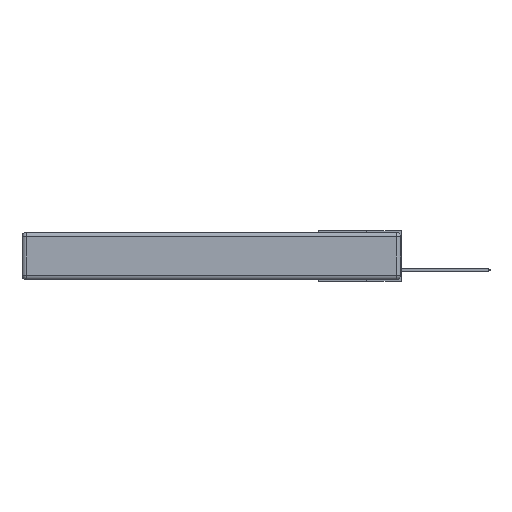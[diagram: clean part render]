
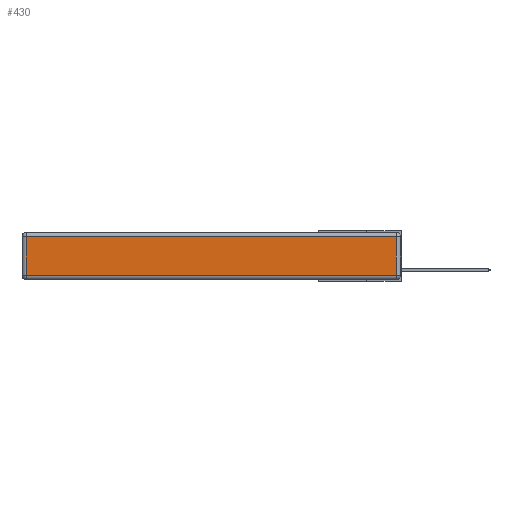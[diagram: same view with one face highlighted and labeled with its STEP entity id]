
A CAD part, left-side view. The second image highlights one B-rep face of the part: STEP entity #430.
In plain terms, the highlighted planar face has unit normal (-1, 0, 0).
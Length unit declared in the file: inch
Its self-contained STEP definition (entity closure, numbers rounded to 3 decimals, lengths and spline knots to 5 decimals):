
#25 = VECTOR ( 'NONE', #13483, 39.37008 ) ;
#243 = CARTESIAN_POINT ( 'NONE',  ( 0., 2.72, -0.343 ) ) ;
#319 = DIRECTION ( 'NONE',  ( 0., 1., 0. ) ) ;
#430 = ADVANCED_FACE ( 'NONE', ( #3738 ), #7658, .T. ) ;
#1101 = ORIENTED_EDGE ( 'NONE', *, *, #12454, .T. ) ;
#1314 = ORIENTED_EDGE ( 'NONE', *, *, #12495, .T. ) ;
#2300 = VERTEX_POINT ( 'NONE', #2312 ) ;
#2312 = CARTESIAN_POINT ( 'NONE',  ( 0., 2.72, -0.03 ) ) ;
#2358 = LINE ( 'NONE', #4114, #3935 ) ;
#2375 = LINE ( 'NONE', #4579, #25 ) ;
#2383 = EDGE_CURVE ( 'NONE', #2300, #3912, #8110, .T. ) ;
#2987 = EDGE_CURVE ( 'NONE', #3912, #9757, #2375, .T. ) ;
#3738 = FACE_OUTER_BOUND ( 'NONE', #11194, .T. ) ;
#3912 = VERTEX_POINT ( 'NONE', #14608 ) ;
#3935 = VECTOR ( 'NONE', #6581, 39.37008 ) ;
#4029 = DIRECTION ( 'NONE',  ( 0., 0., -1. ) ) ;
#4114 = CARTESIAN_POINT ( 'NONE',  ( 0., 0.03, -0.343 ) ) ;
#4579 = CARTESIAN_POINT ( 'NONE',  ( 0., 0., -0.313 ) ) ;
#5947 = VECTOR ( 'NONE', #4029, 39.37008 ) ;
#6581 = DIRECTION ( 'NONE',  ( 0., 0., 1. ) ) ;
#6583 = DIRECTION ( 'NONE',  ( -1., 0., 0. ) ) ;
#7039 = ORIENTED_EDGE ( 'NONE', *, *, #2987, .T. ) ;
#7658 = PLANE ( 'NONE',  #15020 ) ;
#8110 = LINE ( 'NONE', #243, #5947 ) ;
#9052 = CARTESIAN_POINT ( 'NONE',  ( 0., 2.75, -0.03 ) ) ;
#9757 = VERTEX_POINT ( 'NONE', #16175 ) ;
#11194 = EDGE_LOOP ( 'NONE', ( #7039, #1101, #1314, #12809 ) ) ;
#11600 = CARTESIAN_POINT ( 'NONE',  ( 0., 0.03, -0.03 ) ) ;
#11870 = VERTEX_POINT ( 'NONE', #11600 ) ;
#12454 = EDGE_CURVE ( 'NONE', #9757, #11870, #2358, .T. ) ;
#12495 = EDGE_CURVE ( 'NONE', #11870, #2300, #12767, .T. ) ;
#12650 = DIRECTION ( 'NONE',  ( 0., 0., 1. ) ) ;
#12767 = LINE ( 'NONE', #9052, #14311 ) ;
#12775 = CARTESIAN_POINT ( 'NONE',  ( 0., 0., -0.343 ) ) ;
#12809 = ORIENTED_EDGE ( 'NONE', *, *, #2383, .T. ) ;
#13483 = DIRECTION ( 'NONE',  ( 0., -1., 0. ) ) ;
#14311 = VECTOR ( 'NONE', #319, 39.37008 ) ;
#14608 = CARTESIAN_POINT ( 'NONE',  ( 0., 2.72, -0.313 ) ) ;
#15020 = AXIS2_PLACEMENT_3D ( 'NONE', #12775, #6583, #12650 ) ;
#16175 = CARTESIAN_POINT ( 'NONE',  ( 0., 0.03, -0.313 ) ) ;
